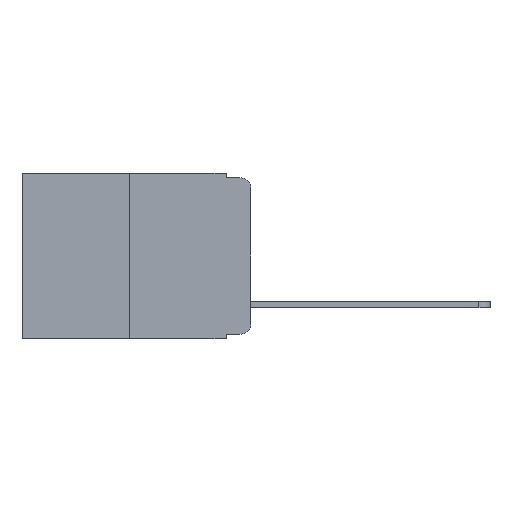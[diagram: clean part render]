
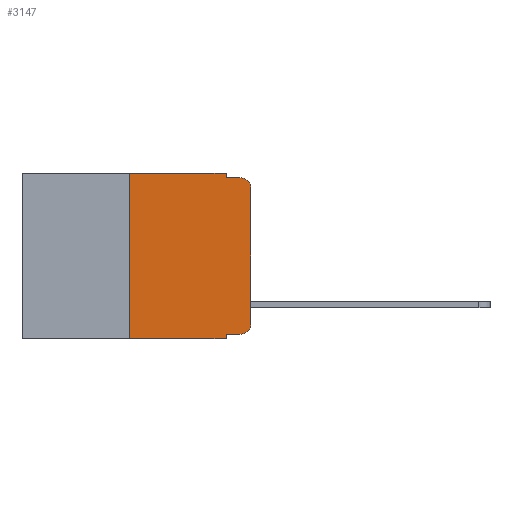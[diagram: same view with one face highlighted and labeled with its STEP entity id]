
A CAD part, left-side view. The second image highlights one B-rep face of the part: STEP entity #3147.
In plain terms, the highlighted planar face has unit normal (-1, 0, 0).
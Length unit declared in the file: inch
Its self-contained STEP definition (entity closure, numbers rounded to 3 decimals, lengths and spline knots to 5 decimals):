
#317 = VERTEX_POINT ( 'NONE', #9929 ) ;
#417 = LINE ( 'NONE', #12029, #5285 ) ;
#560 = EDGE_CURVE ( 'NONE', #1576, #2866, #2210, .T. ) ;
#954 = CARTESIAN_POINT ( 'NONE',  ( 0., 0.051, -0.01 ) ) ;
#1576 = VERTEX_POINT ( 'NONE', #4196 ) ;
#1604 = VERTEX_POINT ( 'NONE', #5093 ) ;
#1947 = LINE ( 'NONE', #9346, #7107 ) ;
#1968 = VERTEX_POINT ( 'NONE', #7947 ) ;
#2000 = AXIS2_PLACEMENT_3D ( 'NONE', #7459, #4695, #4692 ) ;
#2181 = VECTOR ( 'NONE', #3165, 39.37008 ) ;
#2198 = VERTEX_POINT ( 'NONE', #11424 ) ;
#2210 = LINE ( 'NONE', #10105, #2181 ) ;
#2247 = AXIS2_PLACEMENT_3D ( 'NONE', #8724, #8694, #2803 ) ;
#2251 = EDGE_CURVE ( 'NONE', #6013, #1968, #11614, .T. ) ;
#2648 = DIRECTION ( 'NONE',  ( 0., -1., 0. ) ) ;
#2671 = CIRCLE ( 'NONE', #12130, 0.02 ) ;
#2803 = DIRECTION ( 'NONE',  ( 0., 0., -1. ) ) ;
#2866 = VERTEX_POINT ( 'NONE', #954 ) ;
#3047 = VECTOR ( 'NONE', #9468, 39.37008 ) ;
#3147 = ADVANCED_FACE ( 'NONE', ( #5356 ), #8622, .F. ) ;
#3165 = DIRECTION ( 'NONE',  ( 0., 0., -1. ) ) ;
#3313 = CARTESIAN_POINT ( 'NONE',  ( 0., 0.02, -0.03 ) ) ;
#3411 = LINE ( 'NONE', #5251, #8249 ) ;
#4021 = EDGE_LOOP ( 'NONE', ( #5493, #5617, #6255, #8022, #9593, #12056, #10610, #10333, #11857, #10593 ) ) ;
#4196 = CARTESIAN_POINT ( 'NONE',  ( 0., 0.051, 0. ) ) ;
#4205 = VECTOR ( 'NONE', #6406, 39.37008 ) ;
#4345 = DIRECTION ( 'NONE',  ( 0., 0., -1. ) ) ;
#4350 = CARTESIAN_POINT ( 'NONE',  ( 0., 0., -0.03 ) ) ;
#4518 = LINE ( 'NONE', #7299, #4205 ) ;
#4522 = VECTOR ( 'NONE', #10510, 39.37008 ) ;
#4692 = DIRECTION ( 'NONE',  ( 0., 0., -1. ) ) ;
#4695 = DIRECTION ( 'NONE',  ( -1., 0., 0. ) ) ;
#5093 = CARTESIAN_POINT ( 'NONE',  ( 0., 0.051, -0.343 ) ) ;
#5251 = CARTESIAN_POINT ( 'NONE',  ( 0., 0., 0. ) ) ;
#5285 = VECTOR ( 'NONE', #11986, 39.37008 ) ;
#5321 = CARTESIAN_POINT ( 'NONE',  ( 0., 0.25, 0. ) ) ;
#5356 = FACE_OUTER_BOUND ( 'NONE', #4021, .T. ) ;
#5378 = DIRECTION ( 'NONE',  ( 0., 0., 1. ) ) ;
#5493 = ORIENTED_EDGE ( 'NONE', *, *, #11949, .T. ) ;
#5555 = EDGE_CURVE ( 'NONE', #1968, #1576, #5769, .T. ) ;
#5617 = ORIENTED_EDGE ( 'NONE', *, *, #12009, .T. ) ;
#5650 = EDGE_CURVE ( 'NONE', #7207, #1604, #6512, .T. ) ;
#5743 = EDGE_CURVE ( 'NONE', #7207, #7121, #417, .T. ) ;
#5769 = LINE ( 'NONE', #9452, #3047 ) ;
#5902 = CIRCLE ( 'NONE', #2000, 0.02 ) ;
#5989 = EDGE_CURVE ( 'NONE', #7121, #317, #5902, .T. ) ;
#6013 = VERTEX_POINT ( 'NONE', #8536 ) ;
#6241 = DIRECTION ( 'NONE',  ( 0., 0., 1. ) ) ;
#6255 = ORIENTED_EDGE ( 'NONE', *, *, #12129, .F. ) ;
#6406 = DIRECTION ( 'NONE',  ( 0., -1., 0. ) ) ;
#6512 = LINE ( 'NONE', #9334, #4522 ) ;
#6711 = CARTESIAN_POINT ( 'NONE',  ( 0., 0.051, -0.333 ) ) ;
#7107 = VECTOR ( 'NONE', #2648, 39.37008 ) ;
#7121 = VERTEX_POINT ( 'NONE', #11374 ) ;
#7207 = VERTEX_POINT ( 'NONE', #6711 ) ;
#7299 = CARTESIAN_POINT ( 'NONE',  ( 0., 0.051, -0.01 ) ) ;
#7459 = CARTESIAN_POINT ( 'NONE',  ( 0., 0.02, -0.313 ) ) ;
#7947 = CARTESIAN_POINT ( 'NONE',  ( 0., 0.25, 0. ) ) ;
#8022 = ORIENTED_EDGE ( 'NONE', *, *, #560, .F. ) ;
#8249 = VECTOR ( 'NONE', #6241, 39.37008 ) ;
#8536 = CARTESIAN_POINT ( 'NONE',  ( 0., 0.25, -0.343 ) ) ;
#8622 = PLANE ( 'NONE',  #2247 ) ;
#8694 = DIRECTION ( 'NONE',  ( 1., 0., 0. ) ) ;
#8724 = CARTESIAN_POINT ( 'NONE',  ( 0., 0.473, 0. ) ) ;
#9221 = VECTOR ( 'NONE', #5378, 39.37008 ) ;
#9334 = CARTESIAN_POINT ( 'NONE',  ( 0., 0.051, 0. ) ) ;
#9346 = CARTESIAN_POINT ( 'NONE',  ( 0., 0.473, -0.343 ) ) ;
#9452 = CARTESIAN_POINT ( 'NONE',  ( 0., 0.473, 0. ) ) ;
#9468 = DIRECTION ( 'NONE',  ( 0., -1., 0. ) ) ;
#9593 = ORIENTED_EDGE ( 'NONE', *, *, #5555, .F. ) ;
#9820 = DIRECTION ( 'NONE',  ( -1., 0., 0. ) ) ;
#9929 = CARTESIAN_POINT ( 'NONE',  ( 0., 0., -0.313 ) ) ;
#10105 = CARTESIAN_POINT ( 'NONE',  ( 0., 0.051, 0. ) ) ;
#10324 = VERTEX_POINT ( 'NONE', #4350 ) ;
#10333 = ORIENTED_EDGE ( 'NONE', *, *, #5650, .F. ) ;
#10510 = DIRECTION ( 'NONE',  ( 0., 0., -1. ) ) ;
#10593 = ORIENTED_EDGE ( 'NONE', *, *, #5989, .T. ) ;
#10610 = ORIENTED_EDGE ( 'NONE', *, *, #11461, .T. ) ;
#11374 = CARTESIAN_POINT ( 'NONE',  ( 0., 0.02, -0.333 ) ) ;
#11424 = CARTESIAN_POINT ( 'NONE',  ( 0., 0.02, -0.01 ) ) ;
#11461 = EDGE_CURVE ( 'NONE', #6013, #1604, #1947, .T. ) ;
#11614 = LINE ( 'NONE', #5321, #9221 ) ;
#11857 = ORIENTED_EDGE ( 'NONE', *, *, #5743, .T. ) ;
#11949 = EDGE_CURVE ( 'NONE', #317, #10324, #3411, .T. ) ;
#11986 = DIRECTION ( 'NONE',  ( 0., -1., 0. ) ) ;
#12009 = EDGE_CURVE ( 'NONE', #10324, #2198, #2671, .T. ) ;
#12029 = CARTESIAN_POINT ( 'NONE',  ( 0., 0.051, -0.333 ) ) ;
#12056 = ORIENTED_EDGE ( 'NONE', *, *, #2251, .F. ) ;
#12129 = EDGE_CURVE ( 'NONE', #2866, #2198, #4518, .T. ) ;
#12130 = AXIS2_PLACEMENT_3D ( 'NONE', #3313, #9820, #4345 ) ;
